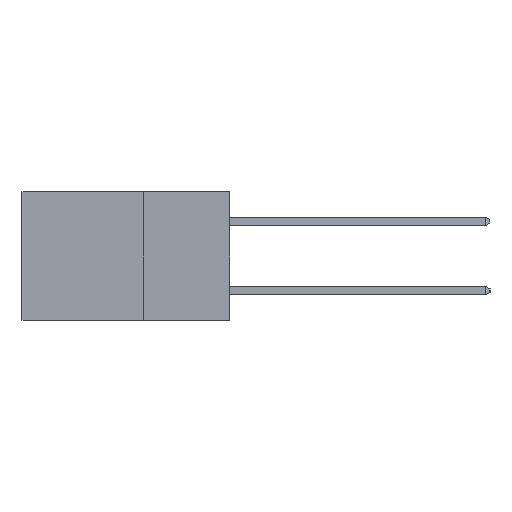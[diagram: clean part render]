
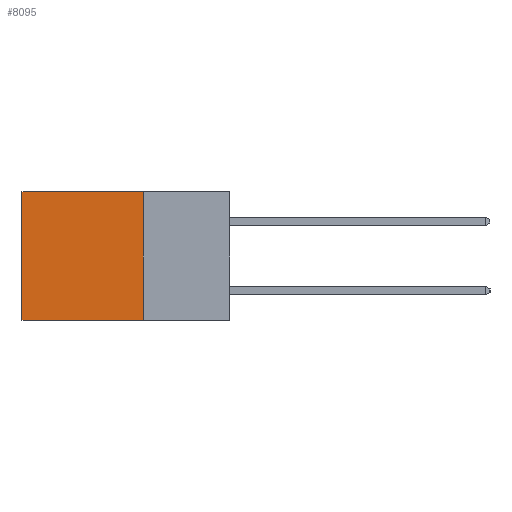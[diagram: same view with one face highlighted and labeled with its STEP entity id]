
A CAD part, left-side view. The second image highlights one B-rep face of the part: STEP entity #8095.
In plain terms, the highlighted planar face has unit normal (-1, 0, 0).
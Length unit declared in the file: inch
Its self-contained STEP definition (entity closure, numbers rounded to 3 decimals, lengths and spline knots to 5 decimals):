
#622 = EDGE_CURVE ( 'NONE', #4995, #6976, #7739, .T. ) ;
#674 = CARTESIAN_POINT ( 'NONE',  ( 0.2615, 0.25, -0.37 ) ) ;
#882 = ORIENTED_EDGE ( 'NONE', *, *, #622, .F. ) ;
#1411 = LINE ( 'NONE', #10912, #3811 ) ;
#1433 = FACE_OUTER_BOUND ( 'NONE', #11186, .T. ) ;
#1558 = ORIENTED_EDGE ( 'NONE', *, *, #8388, .T. ) ;
#2231 = DIRECTION ( 'NONE',  ( 0., 0., -1. ) ) ;
#2356 = DIRECTION ( 'NONE',  ( 0., 1., 0. ) ) ;
#2473 = AXIS2_PLACEMENT_3D ( 'NONE', #7424, #7500, #10032 ) ;
#2780 = LINE ( 'NONE', #5662, #7150 ) ;
#3035 = PLANE ( 'NONE',  #2473 ) ;
#3316 = ORIENTED_EDGE ( 'NONE', *, *, #9065, .T. ) ;
#3607 = VERTEX_POINT ( 'NONE', #9364 ) ;
#3811 = VECTOR ( 'NONE', #5664, 39.37008 ) ;
#4995 = VERTEX_POINT ( 'NONE', #6497 ) ;
#5660 = LINE ( 'NONE', #7522, #8668 ) ;
#5662 = CARTESIAN_POINT ( 'NONE',  ( 0.2615, 0.25, 0. ) ) ;
#5664 = DIRECTION ( 'NONE',  ( 0., 0., -1. ) ) ;
#5907 = CARTESIAN_POINT ( 'NONE',  ( 0.2615, 0.25, 0. ) ) ;
#6497 = CARTESIAN_POINT ( 'NONE',  ( 0.2615, 0.25, -0.37 ) ) ;
#6976 = VERTEX_POINT ( 'NONE', #8875 ) ;
#7150 = VECTOR ( 'NONE', #9947, 39.37008 ) ;
#7217 = VERTEX_POINT ( 'NONE', #5907 ) ;
#7424 = CARTESIAN_POINT ( 'NONE',  ( 0.2615, 0.25, -0.37 ) ) ;
#7443 = EDGE_CURVE ( 'NONE', #7217, #4995, #5660, .T. ) ;
#7500 = DIRECTION ( 'NONE',  ( 1., 0., 0. ) ) ;
#7522 = CARTESIAN_POINT ( 'NONE',  ( 0.2615, 0.25, -0.37 ) ) ;
#7739 = LINE ( 'NONE', #674, #11173 ) ;
#8095 = ADVANCED_FACE ( 'NONE', ( #1433 ), #3035, .F. ) ;
#8388 = EDGE_CURVE ( 'NONE', #7217, #3607, #2780, .T. ) ;
#8668 = VECTOR ( 'NONE', #2231, 39.37008 ) ;
#8851 = ORIENTED_EDGE ( 'NONE', *, *, #7443, .F. ) ;
#8875 = CARTESIAN_POINT ( 'NONE',  ( 0.2615, 0.6, -0.37 ) ) ;
#9065 = EDGE_CURVE ( 'NONE', #3607, #6976, #1411, .T. ) ;
#9364 = CARTESIAN_POINT ( 'NONE',  ( 0.2615, 0.6, 0. ) ) ;
#9947 = DIRECTION ( 'NONE',  ( 0., 1., 0. ) ) ;
#10032 = DIRECTION ( 'NONE',  ( 0., 0., -1. ) ) ;
#10912 = CARTESIAN_POINT ( 'NONE',  ( 0.2615, 0.6, -0.37 ) ) ;
#11173 = VECTOR ( 'NONE', #2356, 39.37008 ) ;
#11186 = EDGE_LOOP ( 'NONE', ( #3316, #882, #8851, #1558 ) ) ;
